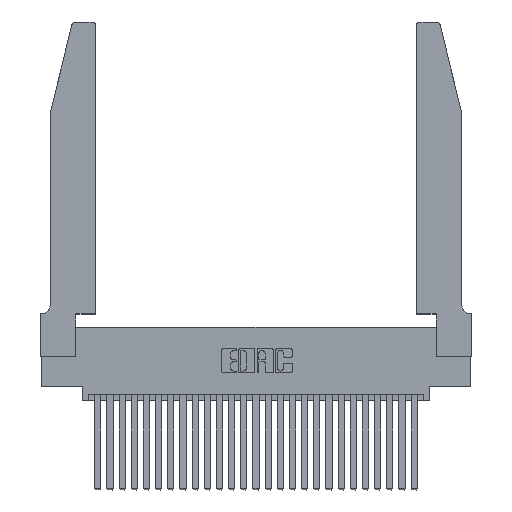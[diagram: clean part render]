
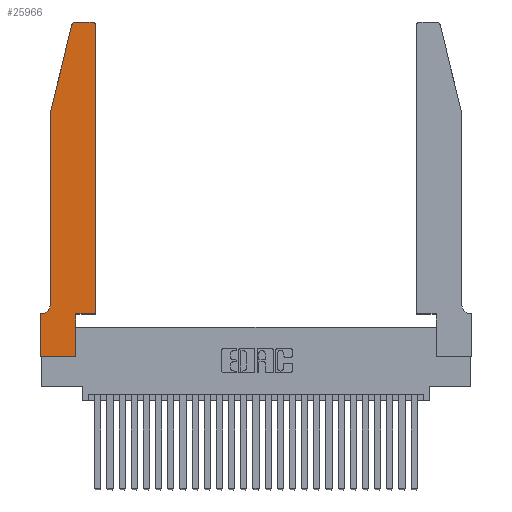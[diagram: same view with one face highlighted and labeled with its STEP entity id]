
A CAD part, top view. The second image highlights one B-rep face of the part: STEP entity #25966.
In plain terms, the highlighted planar face has unit normal (0, 0, 1).
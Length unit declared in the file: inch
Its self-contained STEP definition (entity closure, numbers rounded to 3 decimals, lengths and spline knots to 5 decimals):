
#753 = LINE ( 'NONE', #19998, #21693 ) ;
#1065 = AXIS2_PLACEMENT_3D ( 'NONE', #13063, #27931, #15202 ) ;
#1268 = DIRECTION ( 'NONE',  ( 0., 1., 0. ) ) ;
#1330 = EDGE_CURVE ( 'NONE', #6410, #13806, #15093, .T. ) ;
#1647 = EDGE_CURVE ( 'NONE', #2401, #6410, #13376, .T. ) ;
#1784 = DIRECTION ( 'NONE',  ( -0.239, -0.971, 0. ) ) ;
#2401 = VERTEX_POINT ( 'NONE', #4147 ) ;
#3049 = CARTESIAN_POINT ( 'NONE',  ( 0.0755, 0.42, 0.37 ) ) ;
#4045 = LINE ( 'NONE', #26813, #21824 ) ;
#4147 = CARTESIAN_POINT ( 'NONE',  ( 0.4205, 2.75, 0.37 ) ) ;
#5188 = VERTEX_POINT ( 'NONE', #23446 ) ;
#5306 = VECTOR ( 'NONE', #8074, 39.37008 ) ;
#5669 = VERTEX_POINT ( 'NONE', #22762 ) ;
#5727 = CARTESIAN_POINT ( 'NONE',  ( 0.2605, 2.75, 0.37 ) ) ;
#5747 = CARTESIAN_POINT ( 'NONE',  ( 0., 0., 0.37 ) ) ;
#6291 = CARTESIAN_POINT ( 'NONE',  ( 0.284, 2.75, 0.37 ) ) ;
#6410 = VERTEX_POINT ( 'NONE', #6291 ) ;
#6955 = CARTESIAN_POINT ( 'NONE',  ( 0.284, 2.72, 0.37 ) ) ;
#6996 = ORIENTED_EDGE ( 'NONE', *, *, #1647, .T. ) ;
#7230 = EDGE_CURVE ( 'NONE', #25623, #19035, #24209, .T. ) ;
#7233 = DIRECTION ( 'NONE',  ( 0., 1., 0. ) ) ;
#7350 = CARTESIAN_POINT ( 'NONE',  ( 0.2865, 0.35, 0.37 ) ) ;
#7691 = CIRCLE ( 'NONE', #1065, 0.07 ) ;
#7938 = DIRECTION ( 'NONE',  ( 0., -1., 0. ) ) ;
#7996 = CARTESIAN_POINT ( 'NONE',  ( 0., 0.35, 0.37 ) ) ;
#8074 = DIRECTION ( 'NONE',  ( 0., -1., 0. ) ) ;
#8224 = DIRECTION ( 'NONE',  ( 1., 0., 0. ) ) ;
#8335 = VECTOR ( 'NONE', #9976, 39.37008 ) ;
#9105 = CARTESIAN_POINT ( 'NONE',  ( 0.4505, 0.35, 0.37 ) ) ;
#9113 = DIRECTION ( 'NONE',  ( 1., 0., 0. ) ) ;
#9249 = ORIENTED_EDGE ( 'NONE', *, *, #23060, .T. ) ;
#9463 = EDGE_CURVE ( 'NONE', #9607, #16157, #19004, .T. ) ;
#9607 = VERTEX_POINT ( 'NONE', #23215 ) ;
#9976 = DIRECTION ( 'NONE',  ( -1., 0., 0. ) ) ;
#10417 = DIRECTION ( 'NONE',  ( 0., 0., 1. ) ) ;
#10444 = AXIS2_PLACEMENT_3D ( 'NONE', #19074, #25509, #12781 ) ;
#10616 = ORIENTED_EDGE ( 'NONE', *, *, #17432, .T. ) ;
#11271 = ORIENTED_EDGE ( 'NONE', *, *, #7230, .T. ) ;
#11448 = LINE ( 'NONE', #5747, #22062 ) ;
#11572 = CARTESIAN_POINT ( 'NONE',  ( 0., 0., 0.37 ) ) ;
#11950 = DIRECTION ( 'NONE',  ( -1., 0., 0. ) ) ;
#12022 = ORIENTED_EDGE ( 'NONE', *, *, #21954, .T. ) ;
#12062 = CIRCLE ( 'NONE', #15120, 0.03 ) ;
#12781 = DIRECTION ( 'NONE',  ( 1., 0., 0. ) ) ;
#13063 = CARTESIAN_POINT ( 'NONE',  ( 0.0055, 0.42, 0.37 ) ) ;
#13376 = LINE ( 'NONE', #5727, #8335 ) ;
#13465 = AXIS2_PLACEMENT_3D ( 'NONE', #6955, #21892, #9113 ) ;
#13806 = VERTEX_POINT ( 'NONE', #24151 ) ;
#15093 = CIRCLE ( 'NONE', #13465, 0.03 ) ;
#15120 = AXIS2_PLACEMENT_3D ( 'NONE', #23139, #10417, #25307 ) ;
#15202 = DIRECTION ( 'NONE',  ( -1., 0., 0. ) ) ;
#15318 = EDGE_CURVE ( 'NONE', #19035, #21160, #753, .T. ) ;
#15407 = ORIENTED_EDGE ( 'NONE', *, *, #17953, .T. ) ;
#16157 = VERTEX_POINT ( 'NONE', #25311 ) ;
#16172 = ORIENTED_EDGE ( 'NONE', *, *, #1330, .T. ) ;
#16200 = EDGE_CURVE ( 'NONE', #13806, #5669, #21453, .T. ) ;
#16990 = EDGE_CURVE ( 'NONE', #21160, #9607, #19085, .T. ) ;
#17082 = ORIENTED_EDGE ( 'NONE', *, *, #9463, .T. ) ;
#17189 = VERTEX_POINT ( 'NONE', #7996 ) ;
#17432 = EDGE_CURVE ( 'NONE', #17738, #5188, #7691, .T. ) ;
#17738 = VERTEX_POINT ( 'NONE', #3049 ) ;
#17900 = FACE_OUTER_BOUND ( 'NONE', #21810, .T. ) ;
#17953 = EDGE_CURVE ( 'NONE', #16157, #2401, #12062, .T. ) ;
#18324 = VECTOR ( 'NONE', #1268, 39.37008 ) ;
#18406 = VECTOR ( 'NONE', #26172, 39.37008 ) ;
#18575 = VECTOR ( 'NONE', #8224, 39.37008 ) ;
#19004 = LINE ( 'NONE', #20696, #18324 ) ;
#19035 = VERTEX_POINT ( 'NONE', #24061 ) ;
#19074 = CARTESIAN_POINT ( 'NONE',  ( 0., 0.35, 0.37 ) ) ;
#19085 = LINE ( 'NONE', #9105, #18406 ) ;
#19595 = ORIENTED_EDGE ( 'NONE', *, *, #16200, .T. ) ;
#19998 = CARTESIAN_POINT ( 'NONE',  ( 0.2865, 0.35, 0.37 ) ) ;
#20696 = CARTESIAN_POINT ( 'NONE',  ( 0.4505, 0.35, 0.37 ) ) ;
#20852 = CARTESIAN_POINT ( 'NONE',  ( 0.0755, 2., 0.37 ) ) ;
#21123 = PLANE ( 'NONE',  #10444 ) ;
#21160 = VERTEX_POINT ( 'NONE', #7350 ) ;
#21453 = LINE ( 'NONE', #27357, #26436 ) ;
#21693 = VECTOR ( 'NONE', #7233, 39.37008 ) ;
#21810 = EDGE_LOOP ( 'NONE', ( #6996, #16172, #19595, #24748, #10616, #12022, #9249, #11271, #25730, #25554, #17082, #15407 ) ) ;
#21824 = VECTOR ( 'NONE', #11950, 39.37008 ) ;
#21892 = DIRECTION ( 'NONE',  ( 0., 0., 1. ) ) ;
#21954 = EDGE_CURVE ( 'NONE', #5188, #17189, #4045, .T. ) ;
#22062 = VECTOR ( 'NONE', #7938, 39.37008 ) ;
#22359 = LINE ( 'NONE', #20852, #5306 ) ;
#22762 = CARTESIAN_POINT ( 'NONE',  ( 0.0755, 2., 0.37 ) ) ;
#23060 = EDGE_CURVE ( 'NONE', #17189, #25623, #11448, .T. ) ;
#23139 = CARTESIAN_POINT ( 'NONE',  ( 0.4205, 2.72, 0.37 ) ) ;
#23215 = CARTESIAN_POINT ( 'NONE',  ( 0.4505, 0.35, 0.37 ) ) ;
#23446 = CARTESIAN_POINT ( 'NONE',  ( 0.0055, 0.35, 0.37 ) ) ;
#23760 = EDGE_CURVE ( 'NONE', #5669, #17738, #22359, .T. ) ;
#24061 = CARTESIAN_POINT ( 'NONE',  ( 0.2865, 0., 0.37 ) ) ;
#24151 = CARTESIAN_POINT ( 'NONE',  ( 0.25487, 2.72718, 0.37 ) ) ;
#24209 = LINE ( 'NONE', #27338, #18575 ) ;
#24748 = ORIENTED_EDGE ( 'NONE', *, *, #23760, .T. ) ;
#25307 = DIRECTION ( 'NONE',  ( 1., 0., 0. ) ) ;
#25311 = CARTESIAN_POINT ( 'NONE',  ( 0.4505, 2.72, 0.37 ) ) ;
#25509 = DIRECTION ( 'NONE',  ( 0., 0., 1. ) ) ;
#25554 = ORIENTED_EDGE ( 'NONE', *, *, #16990, .T. ) ;
#25623 = VERTEX_POINT ( 'NONE', #11572 ) ;
#25730 = ORIENTED_EDGE ( 'NONE', *, *, #15318, .T. ) ;
#25966 = ADVANCED_FACE ( 'NONE', ( #17900 ), #21123, .T. ) ;
#26172 = DIRECTION ( 'NONE',  ( 1., 0., 0. ) ) ;
#26436 = VECTOR ( 'NONE', #1784, 39.37008 ) ;
#26813 = CARTESIAN_POINT ( 'NONE',  ( 0.0755, 0.35, 0.37 ) ) ;
#27338 = CARTESIAN_POINT ( 'NONE',  ( 0., 0., 0.37 ) ) ;
#27357 = CARTESIAN_POINT ( 'NONE',  ( 0.0755, 2., 0.37 ) ) ;
#27931 = DIRECTION ( 'NONE',  ( 0., 0., -1. ) ) ;
